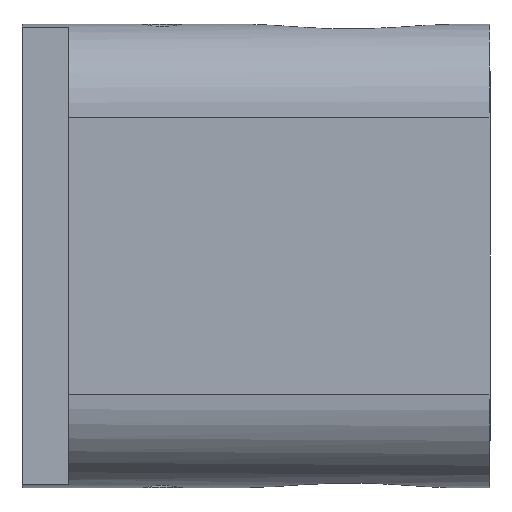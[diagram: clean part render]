
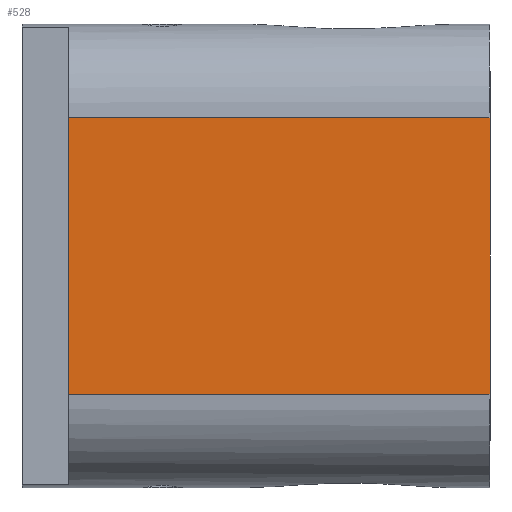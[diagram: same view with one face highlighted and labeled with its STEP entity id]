
A CAD part, left-side view. The second image highlights one B-rep face of the part: STEP entity #528.
In plain terms, the highlighted planar face has unit normal (-1, 0, 0).
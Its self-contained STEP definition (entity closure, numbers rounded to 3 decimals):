
#113=CARTESIAN_POINT('',(-11.,12.,-5.9));
#114=VERTEX_POINT('',#113);
#122=CARTESIAN_POINT('',(-11.,12.,5.9));
#123=VERTEX_POINT('',#122);
#124=CARTESIAN_POINT('',(-11.,12.,5.9));
#125=DIRECTION('',(0.0,0.0,-1.0));
#126=VECTOR('',#125,11.8);
#127=LINE('',#124,#126);
#128=EDGE_CURVE('',#123,#114,#127,.T.);
#197=CARTESIAN_POINT('',(-11.0,-6.,5.9));
#198=VERTEX_POINT('',#197);
#199=CARTESIAN_POINT('',(-11.,12.,5.9));
#200=DIRECTION('',(0.0,-1.0,0.0));
#201=VECTOR('',#200,18.);
#202=LINE('',#199,#201);
#203=EDGE_CURVE('',#123,#198,#202,.T.);
#348=CARTESIAN_POINT('',(-11.0,-6.,-5.9));
#349=VERTEX_POINT('',#348);
#357=CARTESIAN_POINT('',(-11.,-6.,-5.9));
#358=DIRECTION('',(0.0,1.0,0.0));
#359=VECTOR('',#358,18.);
#360=LINE('',#357,#359);
#361=EDGE_CURVE('',#349,#114,#360,.T.);
#484=CARTESIAN_POINT('',(-11.0,-6.,-5.9));
#485=DIRECTION('',(0.0,0.0,1.0));
#486=VECTOR('',#485,11.8);
#487=LINE('',#484,#486);
#488=EDGE_CURVE('',#349,#198,#487,.T.);
#517=CARTESIAN_POINT('',(-11.,12.,0.0));
#518=DIRECTION('',(-1.0,0.0,0.0));
#519=DIRECTION('',(0.0,0.0,1.0));
#520=AXIS2_PLACEMENT_3D('',#517,#518,#519);
#521=PLANE('',#520);
#522=ORIENTED_EDGE('',*,*,#128,.T.);
#523=ORIENTED_EDGE('',*,*,#361,.F.);
#524=ORIENTED_EDGE('',*,*,#488,.T.);
#525=ORIENTED_EDGE('',*,*,#203,.F.);
#526=EDGE_LOOP('',(#522,#523,#524,#525));
#527=FACE_OUTER_BOUND('',#526,.T.);
#528=ADVANCED_FACE('',(#527),#521,.T.);
